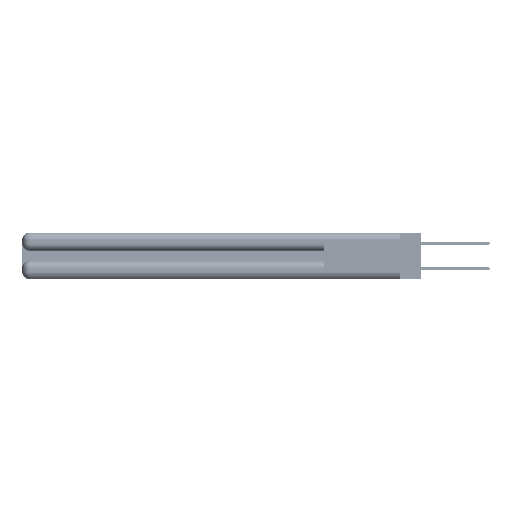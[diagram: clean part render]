
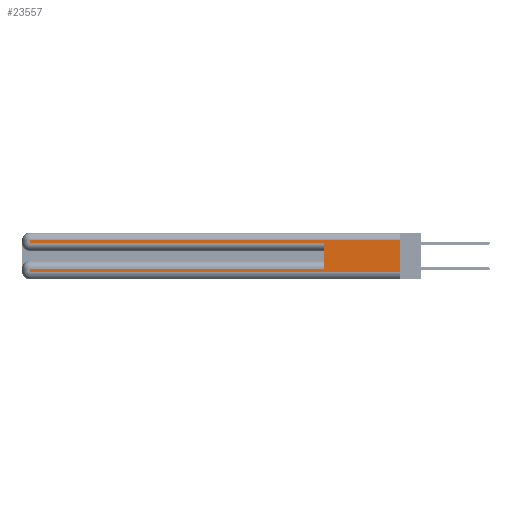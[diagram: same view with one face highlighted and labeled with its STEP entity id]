
A CAD part, left-side view. The second image highlights one B-rep face of the part: STEP entity #23557.
In plain terms, the highlighted planar face has unit normal (-1, 0, 0).
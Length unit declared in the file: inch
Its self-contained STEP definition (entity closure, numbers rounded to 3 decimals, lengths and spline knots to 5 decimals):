
#240 = DIRECTION ( 'NONE',  ( 0., 0., -1. ) ) ;
#1799 = CARTESIAN_POINT ( 'NONE',  ( 0., 0.6, 0.285 ) ) ;
#2455 = VERTEX_POINT ( 'NONE', #1799 ) ;
#3274 = DIRECTION ( 'NONE',  ( 0., 0., -1. ) ) ;
#4323 = ORIENTED_EDGE ( 'NONE', *, *, #54244, .T. ) ;
#4596 = LINE ( 'NONE', #33066, #15819 ) ;
#6330 = DIRECTION ( 'NONE',  ( 0., 0., 1. ) ) ;
#6611 = VECTOR ( 'NONE', #11009, 39.37008 ) ;
#6777 = CARTESIAN_POINT ( 'NONE',  ( 0., 0., 0.31 ) ) ;
#6884 = VECTOR ( 'NONE', #8836, 39.37008 ) ;
#8264 = VERTEX_POINT ( 'NONE', #36999 ) ;
#8836 = DIRECTION ( 'NONE',  ( 0., 1., 0. ) ) ;
#9213 = VERTEX_POINT ( 'NONE', #40915 ) ;
#9397 = CARTESIAN_POINT ( 'NONE',  ( 0., 0., 0.37 ) ) ;
#9590 = CARTESIAN_POINT ( 'NONE',  ( 0., 0., 0.06 ) ) ;
#10086 = CARTESIAN_POINT ( 'NONE',  ( 0., 0., 0.06 ) ) ;
#11009 = DIRECTION ( 'NONE',  ( 0., 0., -1. ) ) ;
#11435 = EDGE_CURVE ( 'NONE', #9213, #2455, #48962, .T. ) ;
#12578 = CARTESIAN_POINT ( 'NONE',  ( 0., 0., 0.285 ) ) ;
#14036 = LINE ( 'NONE', #56132, #42000 ) ;
#15750 = EDGE_CURVE ( 'NONE', #22607, #55947, #14036, .T. ) ;
#15819 = VECTOR ( 'NONE', #6330, 39.37008 ) ;
#17454 = ORIENTED_EDGE ( 'NONE', *, *, #15750, .T. ) ;
#18603 = CARTESIAN_POINT ( 'NONE',  ( 0., 2.94, 0.31 ) ) ;
#20185 = EDGE_CURVE ( 'NONE', #30674, #43114, #50593, .T. ) ;
#21016 = CARTESIAN_POINT ( 'NONE',  ( 0., 0., 0.37 ) ) ;
#21617 = ORIENTED_EDGE ( 'NONE', *, *, #23131, .F. ) ;
#22607 = VERTEX_POINT ( 'NONE', #6777 ) ;
#23131 = EDGE_CURVE ( 'NONE', #8264, #2455, #4596, .T. ) ;
#23557 = ADVANCED_FACE ( 'NONE', ( #27626 ), #57605, .F. ) ;
#24329 = EDGE_CURVE ( 'NONE', #22607, #35331, #53348, .T. ) ;
#25495 = DIRECTION ( 'NONE',  ( 0., 0., -1. ) ) ;
#27323 = VECTOR ( 'NONE', #40830, 39.37008 ) ;
#27626 = FACE_OUTER_BOUND ( 'NONE', #38912, .T. ) ;
#29988 = DIRECTION ( 'NONE',  ( 0., 1., 0. ) ) ;
#30674 = VERTEX_POINT ( 'NONE', #55630 ) ;
#32822 = LINE ( 'NONE', #55965, #50970 ) ;
#33066 = CARTESIAN_POINT ( 'NONE',  ( 0., 0.6, 0.145 ) ) ;
#35331 = VERTEX_POINT ( 'NONE', #10086 ) ;
#36999 = CARTESIAN_POINT ( 'NONE',  ( 0., 0.6, 0.085 ) ) ;
#38818 = AXIS2_PLACEMENT_3D ( 'NONE', #9397, #49226, #240 ) ;
#38912 = EDGE_LOOP ( 'NONE', ( #43958, #17454, #46927, #45260, #21617, #4323, #47683, #40217 ) ) ;
#40217 = ORIENTED_EDGE ( 'NONE', *, *, #49080, .T. ) ;
#40830 = DIRECTION ( 'NONE',  ( 0., -1., 0. ) ) ;
#40915 = CARTESIAN_POINT ( 'NONE',  ( 0., 2.94, 0.285 ) ) ;
#42000 = VECTOR ( 'NONE', #29988, 39.37008 ) ;
#42277 = CARTESIAN_POINT ( 'NONE',  ( 0., 2.94, 0.37 ) ) ;
#43114 = VERTEX_POINT ( 'NONE', #48647 ) ;
#43958 = ORIENTED_EDGE ( 'NONE', *, *, #24329, .F. ) ;
#45260 = ORIENTED_EDGE ( 'NONE', *, *, #11435, .T. ) ;
#45325 = LINE ( 'NONE', #53546, #6884 ) ;
#46927 = ORIENTED_EDGE ( 'NONE', *, *, #53340, .T. ) ;
#47388 = VECTOR ( 'NONE', #57453, 39.37008 ) ;
#47683 = ORIENTED_EDGE ( 'NONE', *, *, #20185, .T. ) ;
#48647 = CARTESIAN_POINT ( 'NONE',  ( 0., 2.94, 0.06 ) ) ;
#48962 = LINE ( 'NONE', #12578, #47388 ) ;
#49080 = EDGE_CURVE ( 'NONE', #43114, #35331, #51060, .T. ) ;
#49140 = VECTOR ( 'NONE', #25495, 39.37008 ) ;
#49226 = DIRECTION ( 'NONE',  ( 1., 0., 0. ) ) ;
#50593 = LINE ( 'NONE', #42277, #6611 ) ;
#50970 = VECTOR ( 'NONE', #3274, 39.37008 ) ;
#51060 = LINE ( 'NONE', #9590, #27323 ) ;
#53340 = EDGE_CURVE ( 'NONE', #55947, #9213, #32822, .T. ) ;
#53348 = LINE ( 'NONE', #21016, #49140 ) ;
#53546 = CARTESIAN_POINT ( 'NONE',  ( 0., 0., 0.085 ) ) ;
#54244 = EDGE_CURVE ( 'NONE', #8264, #30674, #45325, .T. ) ;
#55630 = CARTESIAN_POINT ( 'NONE',  ( 0., 2.94, 0.085 ) ) ;
#55947 = VERTEX_POINT ( 'NONE', #18603 ) ;
#55965 = CARTESIAN_POINT ( 'NONE',  ( 0., 2.94, 0.37 ) ) ;
#56132 = CARTESIAN_POINT ( 'NONE',  ( 0., 0., 0.31 ) ) ;
#57453 = DIRECTION ( 'NONE',  ( 0., -1., 0. ) ) ;
#57605 = PLANE ( 'NONE',  #38818 ) ;
